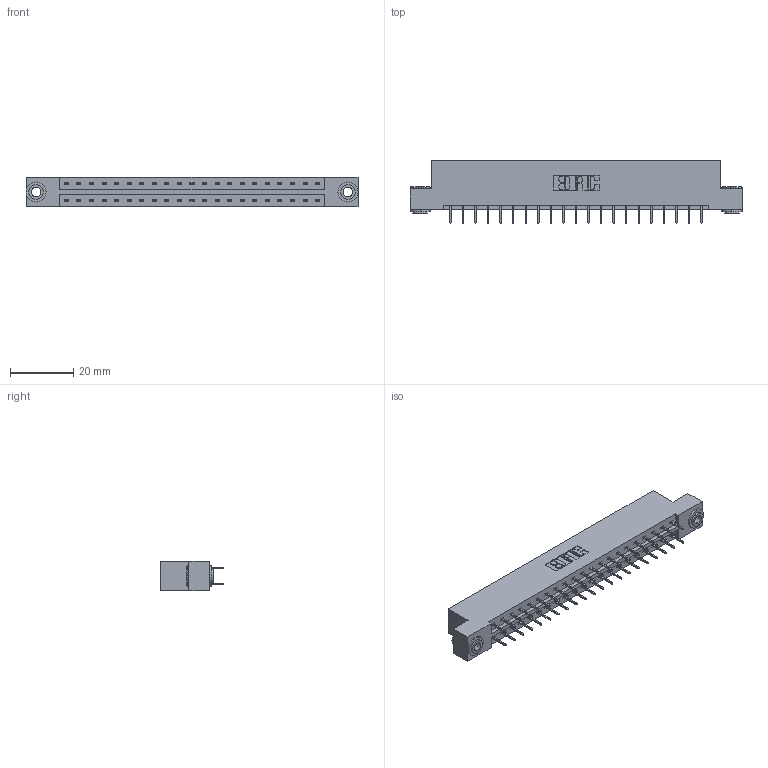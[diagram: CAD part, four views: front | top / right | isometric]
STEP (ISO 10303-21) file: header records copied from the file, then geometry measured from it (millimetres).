
FILE_DESCRIPTION (( 'STEP AP203' ), '1' );
FILE_NAME ('333-042-524-203.STEP', '2018-08-03T18:42:34', ( '' ), ( '' ), 'SwSTEP 2.0', 'SolidWorks 2016', '' );
FILE_SCHEMA (( 'CONFIG_CONTROL_DESIGN' ));
Length unit declared in the file: inch
Products named in the file (4): 345-250-002_345-250-002-102; 333-042-524-203; 333 Part_Flush - .156 Dia - TH; 345-292-001_345-293-124
Assembly tree (45 placements, depth 2):
  333-042-524-203
    333 Part_Flush - .156 Dia - TH
    345-292-001_345-293-124  x42
    345-250-002_345-250-002-102  x2
Bounding box: 104.75 x 19.69 x 9.4 mm (x, y, z)
Volume: 10453.8 mm3; surface area: 12163.4 mm2
Topology: 45 solids, 45 shells, 2504 faces, 7065 edges, 4538 vertices
Faces by surface type: plane 1844, cylinder 652, cone 8
Entity records: 16950 total; most frequent: CARTESIAN_POINT 2809, ORIENTED_EDGE 2738, DIRECTION 2471, EDGE_CURVE 1369, LINE 1221, VECTOR 1221, VERTEX_POINT 906, AXIS2_PLACEMENT_3D 625
